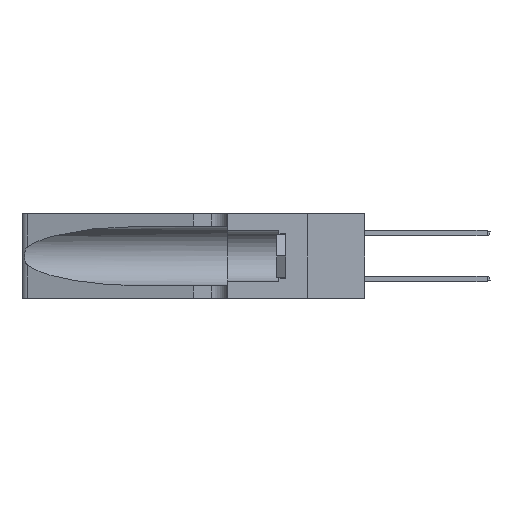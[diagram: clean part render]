
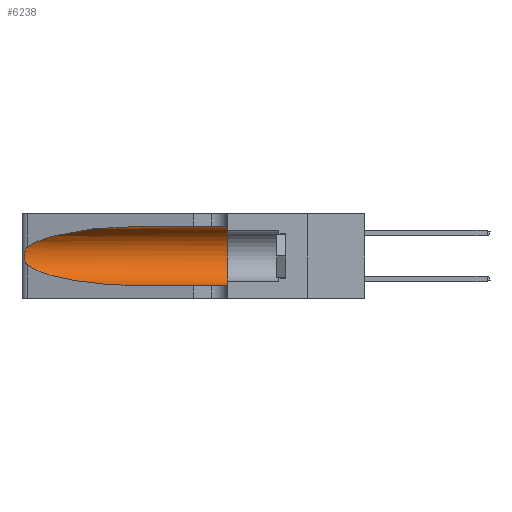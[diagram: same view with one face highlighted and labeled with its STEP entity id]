
A CAD part, left-side view. The second image highlights one B-rep face of the part: STEP entity #6238.
In plain terms, the highlighted cylindrical face has radius 3.308 mm (diameter 6.617 mm), a partial arc.
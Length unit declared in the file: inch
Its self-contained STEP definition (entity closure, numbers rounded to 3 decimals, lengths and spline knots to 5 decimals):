
#1970 = CARTESIAN_POINT ( 'NONE',  ( 0.25487, 1.22718, 0.22369 ) ) ;
#2153 = VERTEX_POINT ( 'NONE', #3931 ) ;
#2309 = CARTESIAN_POINT ( 'NONE',  ( 0.25555, 1.22993, 0.14849 ) ) ;
#3931 = CARTESIAN_POINT ( 'NONE',  ( 0.1305, 0.35, 0.31525 ) ) ;
#4652 = DIRECTION ( 'NONE',  ( 0., -1., 0. ) ) ;
#5669 = CYLINDRICAL_SURFACE ( 'NONE', #23645, 0.13025 ) ;
#6238 = ADVANCED_FACE ( 'NONE', ( #39754 ), #5669, .F. ) ;
#6779 = DIRECTION ( 'NONE',  ( 0., 0., -1. ) ) ;
#8701 = CARTESIAN_POINT ( 'NONE',  ( 0.25787, 1.23484, 0.2124 ) ) ;
#8931 = CARTESIAN_POINT ( 'NONE',  ( 0.1305, 0.72297, 0.31525 ) ) ;
#8937 = ORIENTED_EDGE ( 'NONE', *, *, #14582, .T. ) ;
#9361 = CARTESIAN_POINT ( 'NONE',  ( 0.18966, 0.96281, 0.05475 ) ) ;
#9571 = VERTEX_POINT ( 'NONE', #1970 ) ;
#10576 = CARTESIAN_POINT ( 'NONE',  ( 0.1305, 0.72297, 0.31525 ) ) ;
#10724 = CARTESIAN_POINT ( 'NONE',  ( 0.1305, 0.35, 0.185 ) ) ;
#11155 = EDGE_CURVE ( 'NONE', #9571, #39089, #33030, .T. ) ;
#11790 = CARTESIAN_POINT ( 'NONE',  ( 0.25555, 1.22994, 0.2215 ) ) ;
#11922 = CARTESIAN_POINT ( 'NONE',  ( 0.26018, 1.23835, 0.19895 ) ) ;
#12206 = AXIS2_PLACEMENT_3D ( 'NONE', #10724, #33191, #13929 ) ;
#12941 = ORIENTED_EDGE ( 'NONE', *, *, #34323, .T. ) ;
#13929 = DIRECTION ( 'NONE',  ( 0., 0., 1. ) ) ;
#14075 = VERTEX_POINT ( 'NONE', #25324 ) ;
#14582 = EDGE_CURVE ( 'NONE', #20722, #9571, #25618, .T. ) ;
#15156 = CARTESIAN_POINT ( 'NONE',  ( 0.26075, 1.23896, 0.178 ) ) ;
#16627 = EDGE_CURVE ( 'NONE', #2153, #14075, #40685, .T. ) ;
#17047 = CARTESIAN_POINT ( 'NONE',  ( 0.25487, 1.22718, 0.14631 ) ) ;
#18224 = VECTOR ( 'NONE', #4652, 39.37008 ) ;
#18442 = CARTESIAN_POINT ( 'NONE',  ( 0.25856, 1.23593, 0.16098 ) ) ;
#18464 = EDGE_CURVE ( 'NONE', #20485, #14075, #22532, .T. ) ;
#18949 = CARTESIAN_POINT ( 'NONE',  ( 0.25487, 1.22718, 0.14631 ) ) ;
#20485 = VERTEX_POINT ( 'NONE', #38309 ) ;
#20722 = VERTEX_POINT ( 'NONE', #10576 ) ;
#21711 = CARTESIAN_POINT ( 'NONE',  ( 0.25639, 1.23186, 0.15144 ) ) ;
#21932 = CARTESIAN_POINT ( 'NONE',  ( 0.25487, 1.22718, 0.22369 ) ) ;
#22218 = CARTESIAN_POINT ( 'NONE',  ( 0.2373, 1.15595, 0.08982 ) ) ;
#22529 =( BOUNDED_CURVE ( )  B_SPLINE_CURVE ( 3, ( #18949, #22218, #9361, #31862 ),
 .UNSPECIFIED., .F., .F. ) 
 B_SPLINE_CURVE_WITH_KNOTS ( ( 4, 4 ),
 ( 3.44316, 4.71239 ),
 .UNSPECIFIED. ) 
 CURVE ( )  GEOMETRIC_REPRESENTATION_ITEM ( )  RATIONAL_B_SPLINE_CURVE ( ( 1., 0.87, 0.87, 1. ) ) 
 REPRESENTATION_ITEM ( '' )  );
#22532 = LINE ( 'NONE', #35424, #30033 ) ;
#22739 = DIRECTION ( 'NONE',  ( 0., -1., 0. ) ) ;
#23645 = AXIS2_PLACEMENT_3D ( 'NONE', #35656, #38867, #6779 ) ;
#24604 = ORIENTED_EDGE ( 'NONE', *, *, #27091, .F. ) ;
#24876 = CARTESIAN_POINT ( 'NONE',  ( 0.18966, 0.96281, 0.31525 ) ) ;
#24931 = CARTESIAN_POINT ( 'NONE',  ( 0.25487, 1.22718, 0.14631 ) ) ;
#25324 = CARTESIAN_POINT ( 'NONE',  ( 0.1305, 0.35, 0.05475 ) ) ;
#25618 =( BOUNDED_CURVE ( )  B_SPLINE_CURVE ( 3, ( #8931, #24876, #41006, #21932 ),
 .UNSPECIFIED., .F., .T. ) 
 B_SPLINE_CURVE_WITH_KNOTS ( ( 4, 4 ),
 ( 1.5708, 2.84003 ),
 .UNSPECIFIED. ) 
 CURVE ( )  GEOMETRIC_REPRESENTATION_ITEM ( )  RATIONAL_B_SPLINE_CURVE ( ( 1., 0.87, 0.87, 1. ) ) 
 REPRESENTATION_ITEM ( '' )  );
#26783 = LINE ( 'NONE', #30269, #18224 ) ;
#27091 = EDGE_CURVE ( 'NONE', #20722, #2153, #26783, .T. ) ;
#27444 = EDGE_LOOP ( 'NONE', ( #8937, #28112, #12941, #30094, #32090, #24604 ) ) ;
#28024 = CARTESIAN_POINT ( 'NONE',  ( 0.25639, 1.23184, 0.21858 ) ) ;
#28112 = ORIENTED_EDGE ( 'NONE', *, *, #11155, .T. ) ;
#30033 = VECTOR ( 'NONE', #22739, 39.37008 ) ;
#30094 = ORIENTED_EDGE ( 'NONE', *, *, #18464, .T. ) ;
#30269 = CARTESIAN_POINT ( 'NONE',  ( 0.1305, 1.61858, 0.31525 ) ) ;
#31207 = CARTESIAN_POINT ( 'NONE',  ( 0.25854, 1.2359, 0.20912 ) ) ;
#31862 = CARTESIAN_POINT ( 'NONE',  ( 0.1305, 0.72297, 0.05475 ) ) ;
#32090 = ORIENTED_EDGE ( 'NONE', *, *, #16627, .F. ) ;
#33030 = B_SPLINE_CURVE_WITH_KNOTS ( 'NONE', 3,
 ( #34269, #11790, #28024, #8701, #31207, #11922, #34412, #15156, #37590, #18442, #40798, #21711, #2309, #24931 ),
 .UNSPECIFIED., .F., .F.,
 ( 4, 2, 2, 2, 2, 2, 4 ),
 ( 0., 0.00027, 0.00053, 0.00107, 0.0016, 0.00187, 0.00214 ),
 .UNSPECIFIED. ) ;
#33191 = DIRECTION ( 'NONE',  ( 0., 1., 0. ) ) ;
#34269 = CARTESIAN_POINT ( 'NONE',  ( 0.25487, 1.22718, 0.22369 ) ) ;
#34323 = EDGE_CURVE ( 'NONE', #39089, #20485, #22529, .T. ) ;
#34412 = CARTESIAN_POINT ( 'NONE',  ( 0.26075, 1.23896, 0.19203 ) ) ;
#35424 = CARTESIAN_POINT ( 'NONE',  ( 0.1305, 1.61858, 0.05475 ) ) ;
#35656 = CARTESIAN_POINT ( 'NONE',  ( 0.1305, 1.61858, 0.185 ) ) ;
#37590 = CARTESIAN_POINT ( 'NONE',  ( 0.26017, 1.23833, 0.17102 ) ) ;
#38309 = CARTESIAN_POINT ( 'NONE',  ( 0.1305, 0.72297, 0.05475 ) ) ;
#38867 = DIRECTION ( 'NONE',  ( 0., -1., 0. ) ) ;
#39089 = VERTEX_POINT ( 'NONE', #17047 ) ;
#39754 = FACE_OUTER_BOUND ( 'NONE', #27444, .T. ) ;
#40685 = CIRCLE ( 'NONE', #12206, 0.13025 ) ;
#40798 = CARTESIAN_POINT ( 'NONE',  ( 0.25789, 1.23486, 0.15765 ) ) ;
#41006 = CARTESIAN_POINT ( 'NONE',  ( 0.2373, 1.15595, 0.28018 ) ) ;
